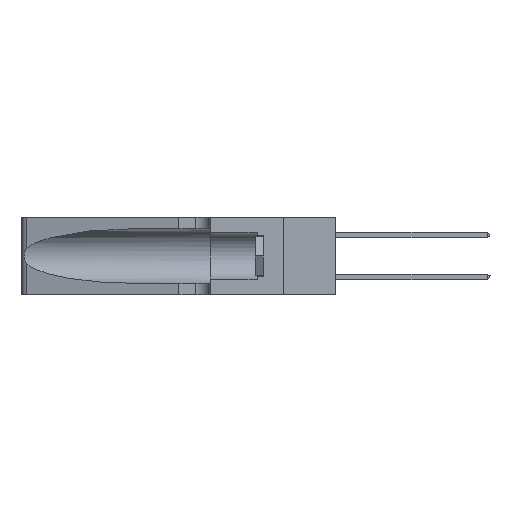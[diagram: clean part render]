
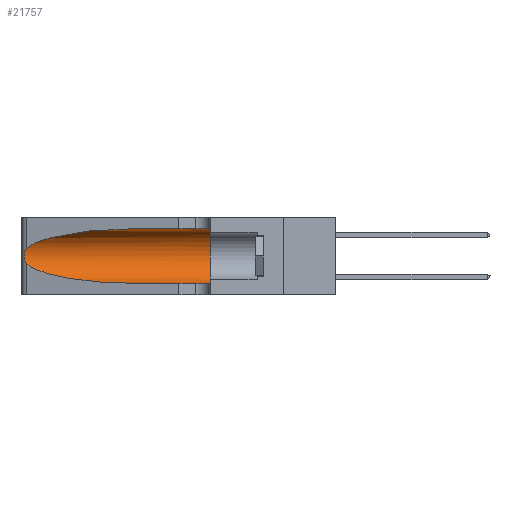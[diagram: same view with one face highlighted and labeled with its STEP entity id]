
A CAD part, left-side view. The second image highlights one B-rep face of the part: STEP entity #21757.
In plain terms, the highlighted cylindrical face has radius 3.308 mm (diameter 6.617 mm), a partial arc.
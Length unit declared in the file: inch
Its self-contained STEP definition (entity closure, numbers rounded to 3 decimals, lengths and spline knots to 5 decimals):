
#437 = CARTESIAN_POINT ( 'NONE',  ( 0.1305, 0.72297, 0.05475 ) ) ;
#734 = CIRCLE ( 'NONE', #7569, 0.13025 ) ;
#2862 = CARTESIAN_POINT ( 'NONE',  ( 0.26075, 1.23896, 0.178 ) ) ;
#3935 = CARTESIAN_POINT ( 'NONE',  ( 0.25487, 1.22718, 0.22369 ) ) ;
#3985 = DIRECTION ( 'NONE',  ( 0., 0., 1. ) ) ;
#4778 = VERTEX_POINT ( 'NONE', #22990 ) ;
#5075 = CARTESIAN_POINT ( 'NONE',  ( 0.25487, 1.22718, 0.22369 ) ) ;
#5986 = VERTEX_POINT ( 'NONE', #6014 ) ;
#6014 = CARTESIAN_POINT ( 'NONE',  ( 0.25487, 1.22718, 0.14631 ) ) ;
#6238 = CARTESIAN_POINT ( 'NONE',  ( 0.26075, 1.23896, 0.19203 ) ) ;
#6282 = B_SPLINE_CURVE_WITH_KNOTS ( 'NONE', 3,
 ( #5075, #29001, #12921, #43196, #23083, #13210, #6238, #2862, #26456, #22669, #27288, #33621, #30687, #13956 ),
 .UNSPECIFIED., .F., .F.,
 ( 4, 2, 2, 2, 2, 2, 4 ),
 ( 0., 0.00027, 0.00053, 0.00107, 0.0016, 0.00187, 0.00214 ),
 .UNSPECIFIED. ) ;
#6329 = EDGE_CURVE ( 'NONE', #4778, #27478, #8959, .T. ) ;
#6661 = DIRECTION ( 'NONE',  ( 0., -1., 0. ) ) ;
#6779 = CYLINDRICAL_SURFACE ( 'NONE', #23412, 0.13025 ) ;
#7211 = CARTESIAN_POINT ( 'NONE',  ( 0.2373, 1.15595, 0.28018 ) ) ;
#7569 = AXIS2_PLACEMENT_3D ( 'NONE', #10979, #34530, #3985 ) ;
#8763 = DIRECTION ( 'NONE',  ( 0., 0., -1. ) ) ;
#8791 = EDGE_CURVE ( 'NONE', #11440, #10672, #30379, .T. ) ;
#8924 = CARTESIAN_POINT ( 'NONE',  ( 0.1305, 1.61858, 0.185 ) ) ;
#8959 = LINE ( 'NONE', #30376, #34799 ) ;
#9781 = VERTEX_POINT ( 'NONE', #38996 ) ;
#10672 = VERTEX_POINT ( 'NONE', #23099 ) ;
#10979 = CARTESIAN_POINT ( 'NONE',  ( 0.1305, 0.35, 0.185 ) ) ;
#11311 = EDGE_CURVE ( 'NONE', #27478, #10672, #734, .T. ) ;
#11440 = VERTEX_POINT ( 'NONE', #437 ) ;
#12921 = CARTESIAN_POINT ( 'NONE',  ( 0.25639, 1.23184, 0.21858 ) ) ;
#13210 = CARTESIAN_POINT ( 'NONE',  ( 0.26018, 1.23835, 0.19895 ) ) ;
#13956 = CARTESIAN_POINT ( 'NONE',  ( 0.25487, 1.22718, 0.14631 ) ) ;
#15003 = EDGE_LOOP ( 'NONE', ( #27469, #19808, #32096, #43433, #43256, #31511 ) ) ;
#15190 = CARTESIAN_POINT ( 'NONE',  ( 0.25487, 1.22718, 0.14631 ) ) ;
#15905 = DIRECTION ( 'NONE',  ( 0., -1., 0. ) ) ;
#16239 = CARTESIAN_POINT ( 'NONE',  ( 0.1305, 0.72297, 0.31525 ) ) ;
#16346 = CARTESIAN_POINT ( 'NONE',  ( 0.1305, 0.35, 0.31525 ) ) ;
#19808 = ORIENTED_EDGE ( 'NONE', *, *, #20899, .T. ) ;
#20899 = EDGE_CURVE ( 'NONE', #9781, #5986, #6282, .T. ) ;
#21757 = ADVANCED_FACE ( 'NONE', ( #38927 ), #6779, .F. ) ;
#21980 = CARTESIAN_POINT ( 'NONE',  ( 0.2373, 1.15595, 0.08982 ) ) ;
#22669 = CARTESIAN_POINT ( 'NONE',  ( 0.25856, 1.23593, 0.16098 ) ) ;
#22990 = CARTESIAN_POINT ( 'NONE',  ( 0.1305, 0.72297, 0.31525 ) ) ;
#23083 = CARTESIAN_POINT ( 'NONE',  ( 0.25854, 1.2359, 0.20912 ) ) ;
#23099 = CARTESIAN_POINT ( 'NONE',  ( 0.1305, 0.35, 0.05475 ) ) ;
#23412 = AXIS2_PLACEMENT_3D ( 'NONE', #8924, #25757, #8763 ) ;
#24952 = EDGE_CURVE ( 'NONE', #5986, #11440, #25795, .T. ) ;
#25757 = DIRECTION ( 'NONE',  ( 0., -1., 0. ) ) ;
#25795 =( BOUNDED_CURVE ( )  B_SPLINE_CURVE ( 3, ( #15190, #21980, #41487, #39379 ),
 .UNSPECIFIED., .F., .F. ) 
 B_SPLINE_CURVE_WITH_KNOTS ( ( 4, 4 ),
 ( 3.44316, 4.71239 ),
 .UNSPECIFIED. ) 
 CURVE ( )  GEOMETRIC_REPRESENTATION_ITEM ( )  RATIONAL_B_SPLINE_CURVE ( ( 1., 0.87, 0.87, 1. ) ) 
 REPRESENTATION_ITEM ( '' )  );
#26049 = CARTESIAN_POINT ( 'NONE',  ( 0.1305, 1.61858, 0.05475 ) ) ;
#26456 = CARTESIAN_POINT ( 'NONE',  ( 0.26017, 1.23833, 0.17102 ) ) ;
#27288 = CARTESIAN_POINT ( 'NONE',  ( 0.25789, 1.23486, 0.15765 ) ) ;
#27333 = EDGE_CURVE ( 'NONE', #4778, #9781, #30318, .T. ) ;
#27469 = ORIENTED_EDGE ( 'NONE', *, *, #27333, .T. ) ;
#27478 = VERTEX_POINT ( 'NONE', #16346 ) ;
#29001 = CARTESIAN_POINT ( 'NONE',  ( 0.25555, 1.22994, 0.2215 ) ) ;
#30318 =( BOUNDED_CURVE ( )  B_SPLINE_CURVE ( 3, ( #16239, #40773, #7211, #3935 ),
 .UNSPECIFIED., .F., .F. ) 
 B_SPLINE_CURVE_WITH_KNOTS ( ( 4, 4 ),
 ( 1.5708, 2.84003 ),
 .UNSPECIFIED. ) 
 CURVE ( )  GEOMETRIC_REPRESENTATION_ITEM ( )  RATIONAL_B_SPLINE_CURVE ( ( 1., 0.87, 0.87, 1. ) ) 
 REPRESENTATION_ITEM ( '' )  );
#30376 = CARTESIAN_POINT ( 'NONE',  ( 0.1305, 1.61858, 0.31525 ) ) ;
#30379 = LINE ( 'NONE', #26049, #30938 ) ;
#30687 = CARTESIAN_POINT ( 'NONE',  ( 0.25555, 1.22993, 0.14849 ) ) ;
#30938 = VECTOR ( 'NONE', #15905, 39.37008 ) ;
#31511 = ORIENTED_EDGE ( 'NONE', *, *, #6329, .F. ) ;
#32096 = ORIENTED_EDGE ( 'NONE', *, *, #24952, .T. ) ;
#33621 = CARTESIAN_POINT ( 'NONE',  ( 0.25639, 1.23186, 0.15144 ) ) ;
#34530 = DIRECTION ( 'NONE',  ( 0., 1., 0. ) ) ;
#34799 = VECTOR ( 'NONE', #6661, 39.37008 ) ;
#38927 = FACE_OUTER_BOUND ( 'NONE', #15003, .T. ) ;
#38996 = CARTESIAN_POINT ( 'NONE',  ( 0.25487, 1.22718, 0.22369 ) ) ;
#39379 = CARTESIAN_POINT ( 'NONE',  ( 0.1305, 0.72297, 0.05475 ) ) ;
#40773 = CARTESIAN_POINT ( 'NONE',  ( 0.18966, 0.96281, 0.31525 ) ) ;
#41487 = CARTESIAN_POINT ( 'NONE',  ( 0.18966, 0.96281, 0.05475 ) ) ;
#43196 = CARTESIAN_POINT ( 'NONE',  ( 0.25787, 1.23484, 0.2124 ) ) ;
#43256 = ORIENTED_EDGE ( 'NONE', *, *, #11311, .F. ) ;
#43433 = ORIENTED_EDGE ( 'NONE', *, *, #8791, .T. ) ;
